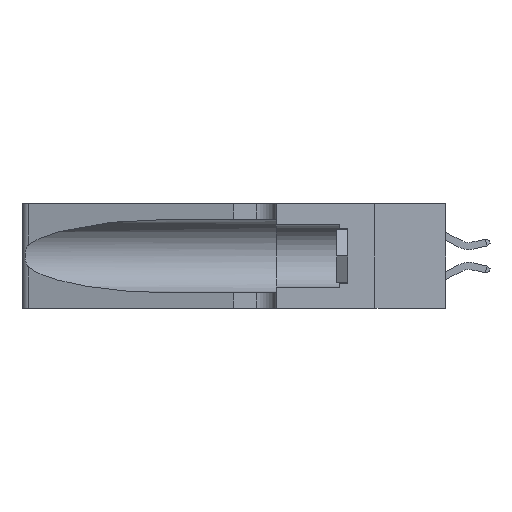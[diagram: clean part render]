
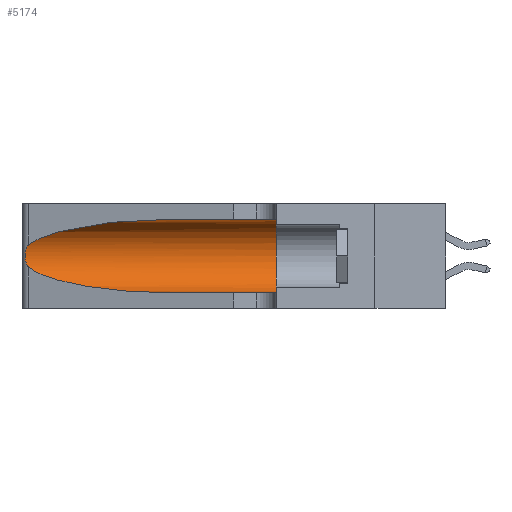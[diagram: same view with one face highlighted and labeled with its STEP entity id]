
A CAD part, left-side view. The second image highlights one B-rep face of the part: STEP entity #5174.
In plain terms, the highlighted cylindrical face has radius 3.308 mm (diameter 6.617 mm), a partial arc.
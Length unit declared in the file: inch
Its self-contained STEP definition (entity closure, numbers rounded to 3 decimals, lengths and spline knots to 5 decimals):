
#598 = CARTESIAN_POINT ( 'NONE',  ( 0.1305, 0.35, 0.31525 ) ) ;
#850 = CARTESIAN_POINT ( 'NONE',  ( 0.25487, 1.22718, 0.22369 ) ) ;
#1753 = CARTESIAN_POINT ( 'NONE',  ( 0.25789, 1.23486, 0.15765 ) ) ;
#2027 = CARTESIAN_POINT ( 'NONE',  ( 0.26075, 1.23896, 0.178 ) ) ;
#2289 = DIRECTION ( 'NONE',  ( 0., 1., 0. ) ) ;
#2592 = FACE_OUTER_BOUND ( 'NONE', #12717, .T. ) ;
#3811 = EDGE_CURVE ( 'NONE', #24605, #33098, #6187, .T. ) ;
#4401 = CARTESIAN_POINT ( 'NONE',  ( 0.1305, 0.72297, 0.05475 ) ) ;
#4565 = VERTEX_POINT ( 'NONE', #598 ) ;
#4610 = ORIENTED_EDGE ( 'NONE', *, *, #26984, .F. ) ;
#4863 = CARTESIAN_POINT ( 'NONE',  ( 0.25487, 1.22718, 0.14631 ) ) ;
#5174 = ADVANCED_FACE ( 'NONE', ( #2592 ), #21637, .F. ) ;
#6187 =( BOUNDED_CURVE ( )  B_SPLINE_CURVE ( 3, ( #36267, #14199, #23807, #33253 ),
 .UNSPECIFIED., .F., .F. ) 
 B_SPLINE_CURVE_WITH_KNOTS ( ( 4, 4 ),
 ( 3.44316, 4.71239 ),
 .UNSPECIFIED. ) 
 CURVE ( )  GEOMETRIC_REPRESENTATION_ITEM ( )  RATIONAL_B_SPLINE_CURVE ( ( 1., 0.87, 0.87, 1. ) ) 
 REPRESENTATION_ITEM ( '' )  );
#6282 = ORIENTED_EDGE ( 'NONE', *, *, #30747, .T. ) ;
#6899 = CARTESIAN_POINT ( 'NONE',  ( 0.1305, 0.72297, 0.31525 ) ) ;
#7552 = CARTESIAN_POINT ( 'NONE',  ( 0.1305, 1.61858, 0.05475 ) ) ;
#7700 = ORIENTED_EDGE ( 'NONE', *, *, #14560, .T. ) ;
#8489 = VECTOR ( 'NONE', #36097, 39.37008 ) ;
#9631 = CARTESIAN_POINT ( 'NONE',  ( 0.2373, 1.15595, 0.28018 ) ) ;
#11722 = CARTESIAN_POINT ( 'NONE',  ( 0.25639, 1.23184, 0.21858 ) ) ;
#11852 = DIRECTION ( 'NONE',  ( 0., 0., 1. ) ) ;
#12717 = EDGE_LOOP ( 'NONE', ( #7700, #6282, #32781, #36362, #4610, #39092 ) ) ;
#13909 = VERTEX_POINT ( 'NONE', #38312 ) ;
#14199 = CARTESIAN_POINT ( 'NONE',  ( 0.2373, 1.15595, 0.08982 ) ) ;
#14291 = CARTESIAN_POINT ( 'NONE',  ( 0.26075, 1.23896, 0.19203 ) ) ;
#14557 = CARTESIAN_POINT ( 'NONE',  ( 0.25555, 1.22994, 0.2215 ) ) ;
#14560 = EDGE_CURVE ( 'NONE', #25974, #29105, #39627, .T. ) ;
#15535 = CARTESIAN_POINT ( 'NONE',  ( 0.25487, 1.22718, 0.14631 ) ) ;
#17439 = CARTESIAN_POINT ( 'NONE',  ( 0.26017, 1.23833, 0.17102 ) ) ;
#17716 = CARTESIAN_POINT ( 'NONE',  ( 0.25854, 1.2359, 0.20912 ) ) ;
#17741 = B_SPLINE_CURVE_WITH_KNOTS ( 'NONE', 3,
 ( #33208, #14557, #11722, #39799, #17716, #21007, #14291, #2027, #17439, #20869, #1753, #36220, #23614, #4863 ),
 .UNSPECIFIED., .F., .F.,
 ( 4, 2, 2, 2, 2, 2, 4 ),
 ( 0., 0.00027, 0.00053, 0.00107, 0.0016, 0.00187, 0.00214 ),
 .UNSPECIFIED. ) ;
#18472 = DIRECTION ( 'NONE',  ( 0., -1., 0. ) ) ;
#20859 = CARTESIAN_POINT ( 'NONE',  ( 0.1305, 1.61858, 0.185 ) ) ;
#20869 = CARTESIAN_POINT ( 'NONE',  ( 0.25856, 1.23593, 0.16098 ) ) ;
#21007 = CARTESIAN_POINT ( 'NONE',  ( 0.26018, 1.23835, 0.19895 ) ) ;
#21377 = CIRCLE ( 'NONE', #36905, 0.13025 ) ;
#21480 = CARTESIAN_POINT ( 'NONE',  ( 0.1305, 1.61858, 0.31525 ) ) ;
#21637 = CYLINDRICAL_SURFACE ( 'NONE', #22523, 0.13025 ) ;
#22523 = AXIS2_PLACEMENT_3D ( 'NONE', #20859, #27209, #36639 ) ;
#23494 = EDGE_CURVE ( 'NONE', #25974, #4565, #32234, .T. ) ;
#23614 = CARTESIAN_POINT ( 'NONE',  ( 0.25555, 1.22993, 0.14849 ) ) ;
#23807 = CARTESIAN_POINT ( 'NONE',  ( 0.18966, 0.96281, 0.05475 ) ) ;
#24605 = VERTEX_POINT ( 'NONE', #15535 ) ;
#25974 = VERTEX_POINT ( 'NONE', #6899 ) ;
#26984 = EDGE_CURVE ( 'NONE', #4565, #13909, #21377, .T. ) ;
#27209 = DIRECTION ( 'NONE',  ( 0., -1., 0. ) ) ;
#28998 = EDGE_CURVE ( 'NONE', #33098, #13909, #36456, .T. ) ;
#29105 = VERTEX_POINT ( 'NONE', #30780 ) ;
#30747 = EDGE_CURVE ( 'NONE', #29105, #24605, #17741, .T. ) ;
#30780 = CARTESIAN_POINT ( 'NONE',  ( 0.25487, 1.22718, 0.22369 ) ) ;
#32234 = LINE ( 'NONE', #21480, #33230 ) ;
#32781 = ORIENTED_EDGE ( 'NONE', *, *, #3811, .T. ) ;
#33098 = VERTEX_POINT ( 'NONE', #4401 ) ;
#33208 = CARTESIAN_POINT ( 'NONE',  ( 0.25487, 1.22718, 0.22369 ) ) ;
#33230 = VECTOR ( 'NONE', #18472, 39.37008 ) ;
#33253 = CARTESIAN_POINT ( 'NONE',  ( 0.1305, 0.72297, 0.05475 ) ) ;
#34449 = CARTESIAN_POINT ( 'NONE',  ( 0.1305, 0.72297, 0.31525 ) ) ;
#36097 = DIRECTION ( 'NONE',  ( 0., -1., 0. ) ) ;
#36220 = CARTESIAN_POINT ( 'NONE',  ( 0.25639, 1.23186, 0.15144 ) ) ;
#36267 = CARTESIAN_POINT ( 'NONE',  ( 0.25487, 1.22718, 0.14631 ) ) ;
#36362 = ORIENTED_EDGE ( 'NONE', *, *, #28998, .T. ) ;
#36456 = LINE ( 'NONE', #7552, #8489 ) ;
#36639 = DIRECTION ( 'NONE',  ( 0., 0., -1. ) ) ;
#36905 = AXIS2_PLACEMENT_3D ( 'NONE', #36924, #2289, #11852 ) ;
#36924 = CARTESIAN_POINT ( 'NONE',  ( 0.1305, 0.35, 0.185 ) ) ;
#37750 = CARTESIAN_POINT ( 'NONE',  ( 0.18966, 0.96281, 0.31525 ) ) ;
#38312 = CARTESIAN_POINT ( 'NONE',  ( 0.1305, 0.35, 0.05475 ) ) ;
#39092 = ORIENTED_EDGE ( 'NONE', *, *, #23494, .F. ) ;
#39627 =( BOUNDED_CURVE ( )  B_SPLINE_CURVE ( 3, ( #34449, #37750, #9631, #850 ),
 .UNSPECIFIED., .F., .T. ) 
 B_SPLINE_CURVE_WITH_KNOTS ( ( 4, 4 ),
 ( 1.5708, 2.84003 ),
 .UNSPECIFIED. ) 
 CURVE ( )  GEOMETRIC_REPRESENTATION_ITEM ( )  RATIONAL_B_SPLINE_CURVE ( ( 1., 0.87, 0.87, 1. ) ) 
 REPRESENTATION_ITEM ( '' )  );
#39799 = CARTESIAN_POINT ( 'NONE',  ( 0.25787, 1.23484, 0.2124 ) ) ;
